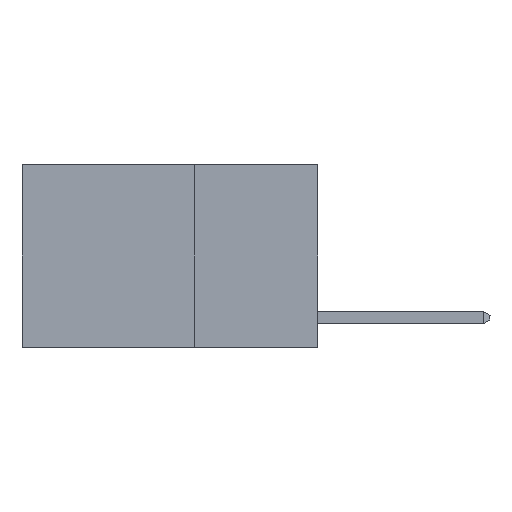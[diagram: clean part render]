
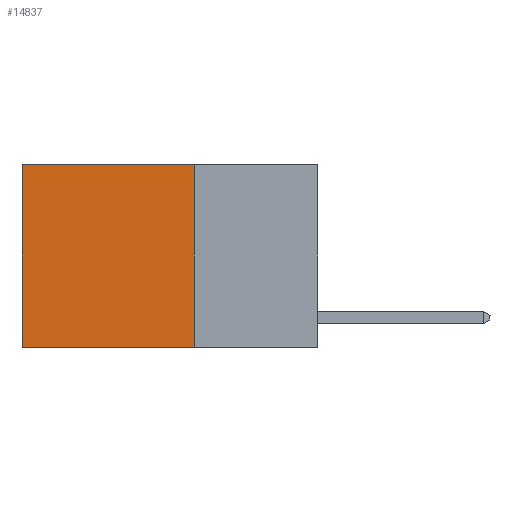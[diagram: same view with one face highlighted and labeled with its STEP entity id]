
A CAD part, left-side view. The second image highlights one B-rep face of the part: STEP entity #14837.
In plain terms, the highlighted planar face has unit normal (-1, 0, 0).
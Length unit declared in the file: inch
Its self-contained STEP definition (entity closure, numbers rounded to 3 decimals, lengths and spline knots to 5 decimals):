
#2434 = VERTEX_POINT ( 'NONE', #4329 ) ;
#2832 = AXIS2_PLACEMENT_3D ( 'NONE', #4039, #27289, #8766 ) ;
#3916 = CARTESIAN_POINT ( 'NONE',  ( 0.2625, 0.25, 0. ) ) ;
#4039 = CARTESIAN_POINT ( 'NONE',  ( 0.2625, 0.25, 0. ) ) ;
#4046 = LINE ( 'NONE', #22722, #17816 ) ;
#4329 = CARTESIAN_POINT ( 'NONE',  ( 0.2625, 0.25, -0.37 ) ) ;
#4588 = VECTOR ( 'NONE', #24273, 39.37008 ) ;
#6169 = VECTOR ( 'NONE', #25868, 39.37008 ) ;
#8303 = EDGE_CURVE ( 'NONE', #10075, #2434, #8670, .T. ) ;
#8374 = CARTESIAN_POINT ( 'NONE',  ( 0.2625, 0.6, -0.37 ) ) ;
#8670 = LINE ( 'NONE', #18048, #9182 ) ;
#8766 = DIRECTION ( 'NONE',  ( 0., 0., -1. ) ) ;
#9182 = VECTOR ( 'NONE', #22485, 39.37008 ) ;
#10075 = VERTEX_POINT ( 'NONE', #3916 ) ;
#13572 = EDGE_CURVE ( 'NONE', #13615, #19577, #18998, .T. ) ;
#13615 = VERTEX_POINT ( 'NONE', #24042 ) ;
#14098 = DIRECTION ( 'NONE',  ( 0., 1., 0. ) ) ;
#14380 = ORIENTED_EDGE ( 'NONE', *, *, #25628, .T. ) ;
#14837 = ADVANCED_FACE ( 'NONE', ( #15372 ), #27141, .F. ) ;
#15128 = ORIENTED_EDGE ( 'NONE', *, *, #8303, .F. ) ;
#15178 = EDGE_LOOP ( 'NONE', ( #17787, #29326, #15128, #14380 ) ) ;
#15372 = FACE_OUTER_BOUND ( 'NONE', #15178, .T. ) ;
#17551 = LINE ( 'NONE', #22132, #4588 ) ;
#17787 = ORIENTED_EDGE ( 'NONE', *, *, #13572, .T. ) ;
#17816 = VECTOR ( 'NONE', #14098, 39.37008 ) ;
#18048 = CARTESIAN_POINT ( 'NONE',  ( 0.2625, 0.25, 0. ) ) ;
#18998 = LINE ( 'NONE', #24187, #6169 ) ;
#19577 = VERTEX_POINT ( 'NONE', #8374 ) ;
#22132 = CARTESIAN_POINT ( 'NONE',  ( 0.2625, 0.25, 0. ) ) ;
#22485 = DIRECTION ( 'NONE',  ( 0., 0., -1. ) ) ;
#22722 = CARTESIAN_POINT ( 'NONE',  ( 0.2625, 0.25, -0.37 ) ) ;
#24042 = CARTESIAN_POINT ( 'NONE',  ( 0.2625, 0.6, 0. ) ) ;
#24187 = CARTESIAN_POINT ( 'NONE',  ( 0.2625, 0.6, 0. ) ) ;
#24273 = DIRECTION ( 'NONE',  ( 0., 1., 0. ) ) ;
#25628 = EDGE_CURVE ( 'NONE', #10075, #13615, #17551, .T. ) ;
#25868 = DIRECTION ( 'NONE',  ( 0., 0., -1. ) ) ;
#27141 = PLANE ( 'NONE',  #2832 ) ;
#27289 = DIRECTION ( 'NONE',  ( 1., 0., 0. ) ) ;
#27932 = EDGE_CURVE ( 'NONE', #2434, #19577, #4046, .T. ) ;
#29326 = ORIENTED_EDGE ( 'NONE', *, *, #27932, .F. ) ;
